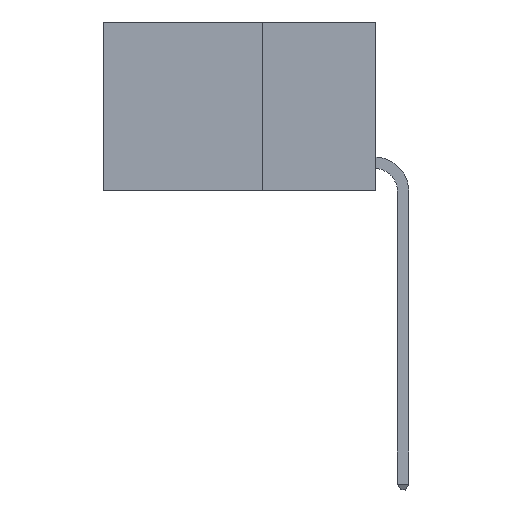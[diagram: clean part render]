
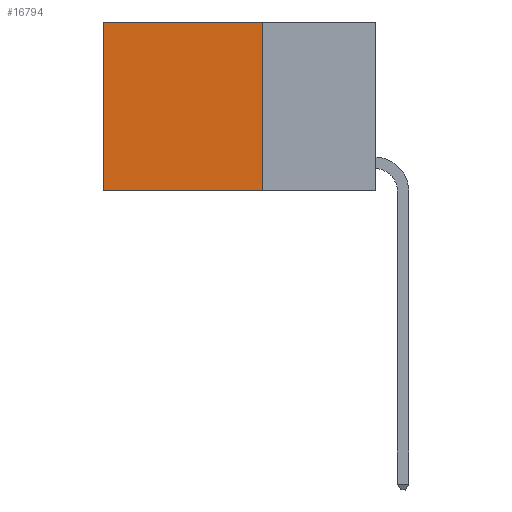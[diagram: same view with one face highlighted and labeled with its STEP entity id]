
A CAD part, left-side view. The second image highlights one B-rep face of the part: STEP entity #16794.
In plain terms, the highlighted planar face has unit normal (-1, 0, 0).
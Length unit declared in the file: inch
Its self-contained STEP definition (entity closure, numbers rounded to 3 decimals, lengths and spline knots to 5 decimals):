
#164 = CARTESIAN_POINT ( 'NONE',  ( 0.2625, 0.6, 0. ) ) ;
#1944 = CARTESIAN_POINT ( 'NONE',  ( 0.2625, 0.25, 0. ) ) ;
#2089 = VECTOR ( 'NONE', #21312, 39.37008 ) ;
#2671 = ORIENTED_EDGE ( 'NONE', *, *, #26516, .F. ) ;
#2704 = VECTOR ( 'NONE', #21455, 39.37008 ) ;
#3016 = VERTEX_POINT ( 'NONE', #164 ) ;
#3099 = CARTESIAN_POINT ( 'NONE',  ( 0.2625, 0.25, -0.37 ) ) ;
#3427 = VECTOR ( 'NONE', #16626, 39.37008 ) ;
#4165 = ORIENTED_EDGE ( 'NONE', *, *, #6167, .F. ) ;
#5221 = EDGE_CURVE ( 'NONE', #7672, #3016, #14802, .T. ) ;
#6167 = EDGE_CURVE ( 'NONE', #7672, #11783, #14144, .T. ) ;
#7100 = CARTESIAN_POINT ( 'NONE',  ( 0.2625, 0.25, 0. ) ) ;
#7672 = VERTEX_POINT ( 'NONE', #23241 ) ;
#8147 = ORIENTED_EDGE ( 'NONE', *, *, #5221, .T. ) ;
#8175 = EDGE_CURVE ( 'NONE', #3016, #11863, #24145, .T. ) ;
#11783 = VERTEX_POINT ( 'NONE', #3099 ) ;
#11863 = VERTEX_POINT ( 'NONE', #23987 ) ;
#12611 = CARTESIAN_POINT ( 'NONE',  ( 0.2625, 0.25, 0. ) ) ;
#12821 = FACE_OUTER_BOUND ( 'NONE', #16474, .T. ) ;
#12856 = DIRECTION ( 'NONE',  ( 1., 0., 0. ) ) ;
#13266 = DIRECTION ( 'NONE',  ( 0., 1., 0. ) ) ;
#13305 = CARTESIAN_POINT ( 'NONE',  ( 0.2625, 0.6, 0. ) ) ;
#14144 = LINE ( 'NONE', #7100, #2704 ) ;
#14802 = LINE ( 'NONE', #12611, #3427 ) ;
#15410 = LINE ( 'NONE', #19184, #20068 ) ;
#16474 = EDGE_LOOP ( 'NONE', ( #24744, #2671, #4165, #8147 ) ) ;
#16626 = DIRECTION ( 'NONE',  ( 0., 1., 0. ) ) ;
#16794 = ADVANCED_FACE ( 'NONE', ( #12821 ), #24771, .F. ) ;
#19184 = CARTESIAN_POINT ( 'NONE',  ( 0.2625, 0.25, -0.37 ) ) ;
#20068 = VECTOR ( 'NONE', #13266, 39.37008 ) ;
#21312 = DIRECTION ( 'NONE',  ( 0., 0., -1. ) ) ;
#21455 = DIRECTION ( 'NONE',  ( 0., 0., -1. ) ) ;
#22860 = AXIS2_PLACEMENT_3D ( 'NONE', #1944, #12856, #26780 ) ;
#23241 = CARTESIAN_POINT ( 'NONE',  ( 0.2625, 0.25, 0. ) ) ;
#23987 = CARTESIAN_POINT ( 'NONE',  ( 0.2625, 0.6, -0.37 ) ) ;
#24145 = LINE ( 'NONE', #13305, #2089 ) ;
#24744 = ORIENTED_EDGE ( 'NONE', *, *, #8175, .T. ) ;
#24771 = PLANE ( 'NONE',  #22860 ) ;
#26516 = EDGE_CURVE ( 'NONE', #11783, #11863, #15410, .T. ) ;
#26780 = DIRECTION ( 'NONE',  ( 0., 0., -1. ) ) ;
